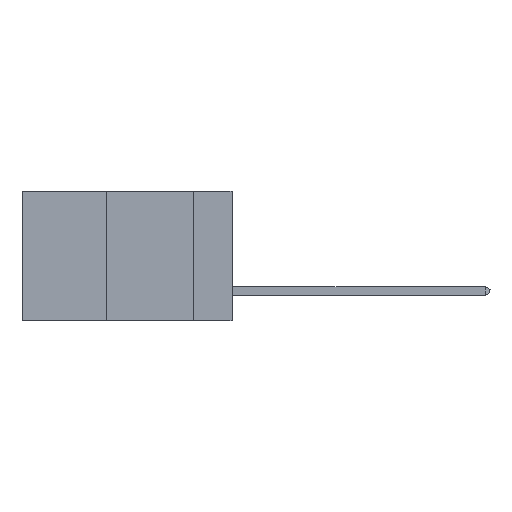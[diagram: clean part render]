
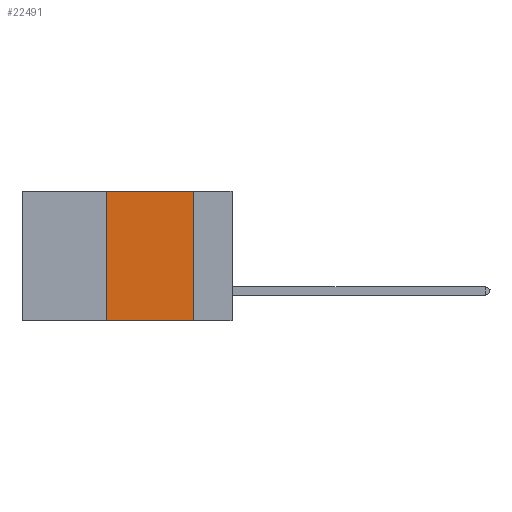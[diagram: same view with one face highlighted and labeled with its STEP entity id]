
A CAD part, left-side view. The second image highlights one B-rep face of the part: STEP entity #22491.
In plain terms, the highlighted planar face has unit normal (-1, 0, 0).
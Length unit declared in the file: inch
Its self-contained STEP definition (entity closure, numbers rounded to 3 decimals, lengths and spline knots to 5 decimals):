
#1097 = VERTEX_POINT ( 'NONE', #18512 ) ;
#1129 = DIRECTION ( 'NONE',  ( 0., 0., 1. ) ) ;
#1276 = AXIS2_PLACEMENT_3D ( 'NONE', #16355, #5857, #20264 ) ;
#4760 = VERTEX_POINT ( 'NONE', #26388 ) ;
#5857 = DIRECTION ( 'NONE',  ( 1., 0., 0. ) ) ;
#11472 = VECTOR ( 'NONE', #1129, 39.37008 ) ;
#12540 = ORIENTED_EDGE ( 'NONE', *, *, #28342, .F. ) ;
#12838 = DIRECTION ( 'NONE',  ( 0., -1., 0. ) ) ;
#14771 = VECTOR ( 'NONE', #14834, 39.37008 ) ;
#14834 = DIRECTION ( 'NONE',  ( 0., -1., 0. ) ) ;
#15921 = LINE ( 'NONE', #42517, #26517 ) ;
#16355 = CARTESIAN_POINT ( 'NONE',  ( 0., 0.6, 0. ) ) ;
#17759 = VERTEX_POINT ( 'NONE', #19640 ) ;
#18512 = CARTESIAN_POINT ( 'NONE',  ( 0., 0.36, 0. ) ) ;
#19640 = CARTESIAN_POINT ( 'NONE',  ( 0., 0.11, -0.37 ) ) ;
#20264 = DIRECTION ( 'NONE',  ( 0., 0., -1. ) ) ;
#20978 = DIRECTION ( 'NONE',  ( 0., 0., -1. ) ) ;
#21318 = VECTOR ( 'NONE', #12838, 39.37008 ) ;
#21874 = CARTESIAN_POINT ( 'NONE',  ( 0., 0.36, -0.37 ) ) ;
#22491 = ADVANCED_FACE ( 'NONE', ( #41393 ), #23206, .F. ) ;
#23206 = PLANE ( 'NONE',  #1276 ) ;
#24261 = CARTESIAN_POINT ( 'NONE',  ( 0., 0.36, 0. ) ) ;
#26388 = CARTESIAN_POINT ( 'NONE',  ( 0., 0.11, 0. ) ) ;
#26517 = VECTOR ( 'NONE', #20978, 39.37008 ) ;
#27824 = EDGE_CURVE ( 'NONE', #42379, #1097, #36169, .T. ) ;
#28052 = ORIENTED_EDGE ( 'NONE', *, *, #37073, .T. ) ;
#28342 = EDGE_CURVE ( 'NONE', #4760, #17759, #15921, .T. ) ;
#28551 = LINE ( 'NONE', #45004, #21318 ) ;
#28653 = EDGE_CURVE ( 'NONE', #1097, #4760, #33888, .T. ) ;
#30910 = ORIENTED_EDGE ( 'NONE', *, *, #28653, .F. ) ;
#32289 = ORIENTED_EDGE ( 'NONE', *, *, #27824, .F. ) ;
#33888 = LINE ( 'NONE', #36326, #14771 ) ;
#36169 = LINE ( 'NONE', #24261, #11472 ) ;
#36326 = CARTESIAN_POINT ( 'NONE',  ( 0., 0.6, 0. ) ) ;
#37073 = EDGE_CURVE ( 'NONE', #42379, #17759, #28551, .T. ) ;
#41393 = FACE_OUTER_BOUND ( 'NONE', #43871, .T. ) ;
#42379 = VERTEX_POINT ( 'NONE', #21874 ) ;
#42517 = CARTESIAN_POINT ( 'NONE',  ( 0., 0.11, 0. ) ) ;
#43871 = EDGE_LOOP ( 'NONE', ( #12540, #30910, #32289, #28052 ) ) ;
#45004 = CARTESIAN_POINT ( 'NONE',  ( 0., 0.6, -0.37 ) ) ;
